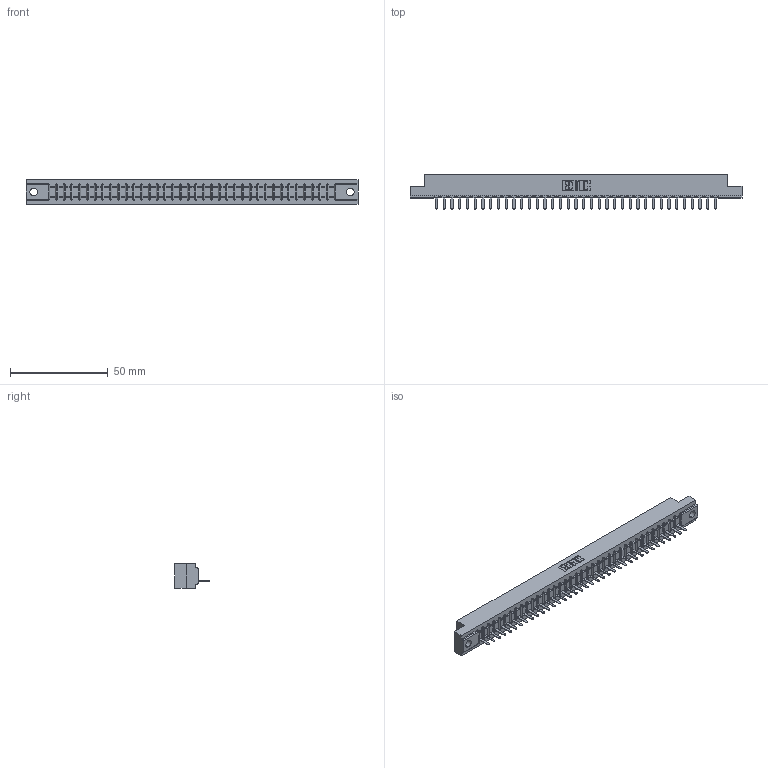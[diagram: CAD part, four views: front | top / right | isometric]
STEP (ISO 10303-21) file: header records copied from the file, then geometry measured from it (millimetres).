
FILE_DESCRIPTION (( 'STEP AP203' ), '1' );
FILE_NAME ('307-037-421-104.STEP', '2020-09-29T04:07:02', ( '' ), ( '' ), 'SwSTEP 2.0', 'SolidWorks 2020', '' );
FILE_SCHEMA (( 'CONFIG_CONTROL_DESIGN' ));
Length unit declared in the file: inch
Products named in the file (3): 307 Part_.156 Dia Mounting Holes; 307-037-421-104; 307-290-002_521
Assembly tree (38 placements, depth 2):
  307-037-421-104
    307 Part_.156 Dia Mounting Holes
    307-290-002_521  x37
Bounding box: 169.62 x 17.42 x 12.7 mm (x, y, z)
Volume: 18010.6 mm3; surface area: 22378.2 mm2
Topology: 38 solids, 38 shells, 2908 faces, 8943 edges, 5858 vertices
Faces by surface type: plane 1749, cylinder 1083, sphere 76
Entity records: 33472 total; most frequent: CARTESIAN_POINT 5650, ORIENTED_EDGE 5638, DIRECTION 5483, EDGE_CURVE 2819, LINE 2165, VECTOR 2165, VERTEX_POINT 1826, AXIS2_PLACEMENT_3D 1659
